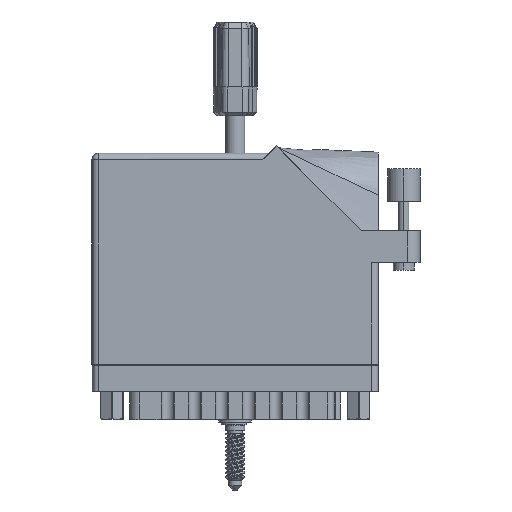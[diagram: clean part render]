
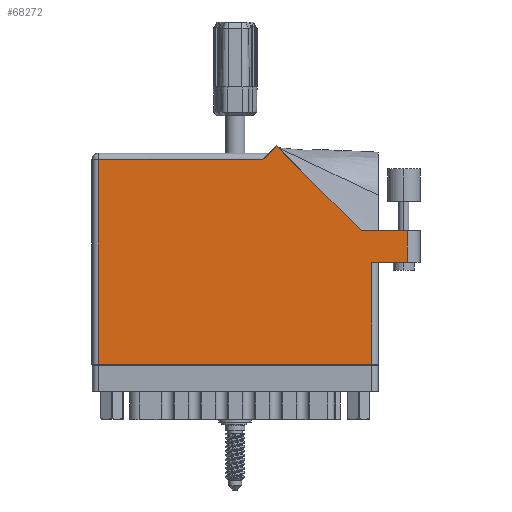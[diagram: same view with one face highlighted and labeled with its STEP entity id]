
A CAD part, front view. The second image highlights one B-rep face of the part: STEP entity #68272.
In plain terms, the highlighted face is planar.
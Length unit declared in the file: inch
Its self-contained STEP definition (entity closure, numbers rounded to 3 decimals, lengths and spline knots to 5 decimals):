
#5899 = CARTESIAN_POINT ( 'NONE',  ( 1.77571, 2.10071, 0. ) ) ;
#6181 = ORIENTED_EDGE ( 'NONE', *, *, #61541, .T. ) ;
#6827 = ORIENTED_EDGE ( 'NONE', *, *, #69487, .T. ) ;
#8311 = DIRECTION ( 'NONE',  ( 0., 1., 0. ) ) ;
#8392 = EDGE_CURVE ( 'NONE', #80822, #73293, #97625, .T. ) ;
#12706 = VERTEX_POINT ( 'NONE', #79529 ) ;
#16954 = EDGE_CURVE ( 'NONE', #74075, #12706, #67198, .T. ) ;
#18537 = VECTOR ( 'NONE', #41178, 39.37008 ) ;
#18796 = LINE ( 'NONE', #48968, #108383 ) ;
#20347 = CARTESIAN_POINT ( 'NONE',  ( 2.755, 0.98, 0. ) ) ;
#20987 = EDGE_CURVE ( 'NONE', #24902, #25187, #18796, .T. ) ;
#21503 = DIRECTION ( 'NONE',  ( 1., 0., 0. ) ) ;
#22751 = AXIS2_PLACEMENT_3D ( 'NONE', #59205, #42917, #41435 ) ;
#24023 = EDGE_CURVE ( 'NONE', #104246, #30892, #108909, .T. ) ;
#24311 = DIRECTION ( 'NONE',  ( -0.707, -0.707, 0. ) ) ;
#24902 = VERTEX_POINT ( 'NONE', #39988 ) ;
#25129 = CARTESIAN_POINT ( 'NONE',  ( 3.03, 1.287, 0. ) ) ;
#25187 = VERTEX_POINT ( 'NONE', #104731 ) ;
#25254 = ORIENTED_EDGE ( 'NONE', *, *, #105558, .T. ) ;
#25485 = ORIENTED_EDGE ( 'NONE', *, *, #16954, .T. ) ;
#28442 = ORIENTED_EDGE ( 'NONE', *, *, #83971, .T. ) ;
#30293 = CARTESIAN_POINT ( 'NONE',  ( 0.062, 1.968, 0. ) ) ;
#30892 = VERTEX_POINT ( 'NONE', #38234 ) ;
#30894 = VERTEX_POINT ( 'NONE', #30293 ) ;
#32371 = CARTESIAN_POINT ( 'NONE',  ( 0., 1.968, 0. ) ) ;
#33200 = VECTOR ( 'NONE', #8311, 39.37008 ) ;
#33223 = ORIENTED_EDGE ( 'NONE', *, *, #8392, .T. ) ;
#33551 = ORIENTED_EDGE ( 'NONE', *, *, #24023, .T. ) ;
#36236 = CARTESIAN_POINT ( 'NONE',  ( 2.58942, 1.287, 0. ) ) ;
#37093 = LINE ( 'NONE', #36236, #58709 ) ;
#38234 = CARTESIAN_POINT ( 'NONE',  ( 1.643, 1.968, 0. ) ) ;
#39733 = VECTOR ( 'NONE', #24311, 39.37008 ) ;
#39988 = CARTESIAN_POINT ( 'NONE',  ( 0.062, 0., 0. ) ) ;
#41178 = DIRECTION ( 'NONE',  ( 0., 1., 0. ) ) ;
#41435 = DIRECTION ( 'NONE',  ( -1., 0., 0. ) ) ;
#42917 = DIRECTION ( 'NONE',  ( 0., 0., -1. ) ) ;
#48968 = CARTESIAN_POINT ( 'NONE',  ( 0., 0., 0. ) ) ;
#49471 = CARTESIAN_POINT ( 'NONE',  ( 2.58942, 1.287, 0. ) ) ;
#54200 = LINE ( 'NONE', #32371, #56927 ) ;
#56927 = VECTOR ( 'NONE', #93368, 39.37008 ) ;
#58709 = VECTOR ( 'NONE', #96885, 39.37008 ) ;
#59205 = CARTESIAN_POINT ( 'NONE',  ( 0., 2.03, 0. ) ) ;
#61541 = EDGE_CURVE ( 'NONE', #30892, #30894, #54200, .T. ) ;
#64164 = EDGE_LOOP ( 'NONE', ( #25485, #6827, #33223, #28442, #33551, #6181, #73397, #102690, #25254 ) ) ;
#66036 = FACE_OUTER_BOUND ( 'NONE', #64164, .T. ) ;
#67198 = LINE ( 'NONE', #20347, #72630 ) ;
#67623 = VECTOR ( 'NONE', #101995, 39.37008 ) ;
#68272 = ADVANCED_FACE ( 'NONE', ( #66036 ), #94832, .F. ) ;
#69487 = EDGE_CURVE ( 'NONE', #12706, #80822, #71370, .T. ) ;
#69879 = CARTESIAN_POINT ( 'NONE',  ( 2.693, 0.98, 0. ) ) ;
#71370 = LINE ( 'NONE', #92719, #18537 ) ;
#71837 = DIRECTION ( 'NONE',  ( -1., 0., 0. ) ) ;
#72630 = VECTOR ( 'NONE', #21503, 39.37008 ) ;
#73293 = VERTEX_POINT ( 'NONE', #49471 ) ;
#73397 = ORIENTED_EDGE ( 'NONE', *, *, #111251, .T. ) ;
#74075 = VERTEX_POINT ( 'NONE', #69879 ) ;
#76206 = CARTESIAN_POINT ( 'NONE',  ( 1.705, 2.03, 0. ) ) ;
#77100 = LINE ( 'NONE', #103119, #67623 ) ;
#79529 = CARTESIAN_POINT ( 'NONE',  ( 3.03, 0.98, 0. ) ) ;
#80822 = VERTEX_POINT ( 'NONE', #25129 ) ;
#81306 = VECTOR ( 'NONE', #71837, 39.37008 ) ;
#83971 = EDGE_CURVE ( 'NONE', #73293, #104246, #37093, .T. ) ;
#86487 = CARTESIAN_POINT ( 'NONE',  ( 2.693, 0.98, 0. ) ) ;
#92719 = CARTESIAN_POINT ( 'NONE',  ( 3.03, 1.287, 0. ) ) ;
#93368 = DIRECTION ( 'NONE',  ( -1., 0., 0. ) ) ;
#94196 = LINE ( 'NONE', #86487, #33200 ) ;
#94832 = PLANE ( 'NONE',  #22751 ) ;
#96885 = DIRECTION ( 'NONE',  ( -0.707, 0.707, 0. ) ) ;
#97625 = LINE ( 'NONE', #112446, #81306 ) ;
#101690 = DIRECTION ( 'NONE',  ( 1., 0., 0. ) ) ;
#101995 = DIRECTION ( 'NONE',  ( 0., -1., 0. ) ) ;
#102690 = ORIENTED_EDGE ( 'NONE', *, *, #20987, .T. ) ;
#103119 = CARTESIAN_POINT ( 'NONE',  ( 0.062, 0., 0. ) ) ;
#104246 = VERTEX_POINT ( 'NONE', #5899 ) ;
#104731 = CARTESIAN_POINT ( 'NONE',  ( 2.693, 0., 0. ) ) ;
#105558 = EDGE_CURVE ( 'NONE', #25187, #74075, #94196, .T. ) ;
#108383 = VECTOR ( 'NONE', #101690, 39.37008 ) ;
#108909 = LINE ( 'NONE', #76206, #39733 ) ;
#111251 = EDGE_CURVE ( 'NONE', #30894, #24902, #77100, .T. ) ;
#112446 = CARTESIAN_POINT ( 'NONE',  ( 3.155, 1.287, 0. ) ) ;
